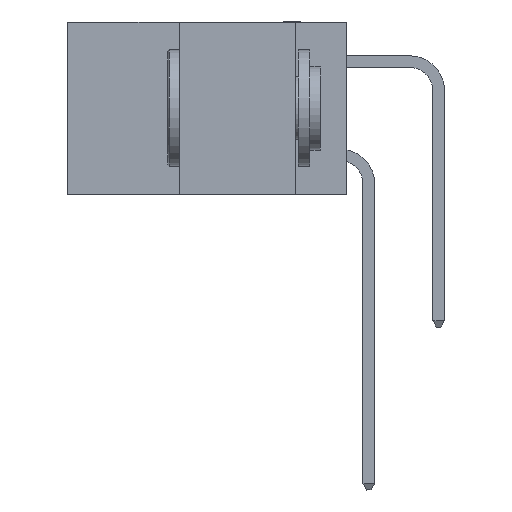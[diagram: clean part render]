
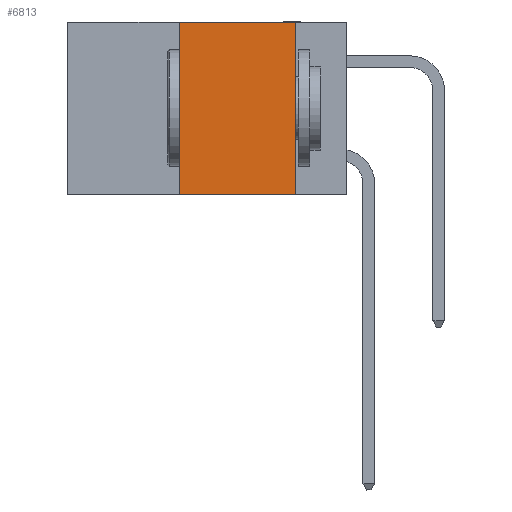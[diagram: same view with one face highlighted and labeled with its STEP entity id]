
A CAD part, left-side view. The second image highlights one B-rep face of the part: STEP entity #6813.
In plain terms, the highlighted planar face has unit normal (-1, 0, 0).
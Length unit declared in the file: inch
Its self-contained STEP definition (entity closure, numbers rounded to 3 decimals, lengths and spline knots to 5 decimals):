
#125 = EDGE_CURVE ( 'NONE', #14238, #33200, #35352, .T. ) ;
#532 = CARTESIAN_POINT ( 'NONE',  ( 0., 0.6, 0. ) ) ;
#647 = DIRECTION ( 'NONE',  ( 0., 0., -1. ) ) ;
#1211 = EDGE_LOOP ( 'NONE', ( #28607, #25209, #31138, #18155 ) ) ;
#2256 = LINE ( 'NONE', #3740, #25788 ) ;
#3740 = CARTESIAN_POINT ( 'NONE',  ( 0., 0.36, 0. ) ) ;
#4098 = EDGE_CURVE ( 'NONE', #16707, #33200, #16321, .T. ) ;
#5903 = VECTOR ( 'NONE', #12400, 39.37008 ) ;
#6072 = PLANE ( 'NONE',  #8083 ) ;
#6355 = DIRECTION ( 'NONE',  ( 0., 0., 1. ) ) ;
#6497 = VECTOR ( 'NONE', #10852, 39.37008 ) ;
#6813 = ADVANCED_FACE ( 'NONE', ( #23195 ), #6072, .F. ) ;
#8083 = AXIS2_PLACEMENT_3D ( 'NONE', #532, #8919, #647 ) ;
#8919 = DIRECTION ( 'NONE',  ( 1., 0., 0. ) ) ;
#10130 = CARTESIAN_POINT ( 'NONE',  ( 0., 0.6, 0. ) ) ;
#10710 = EDGE_CURVE ( 'NONE', #28517, #16707, #28881, .T. ) ;
#10852 = DIRECTION ( 'NONE',  ( 0., 0., -1. ) ) ;
#12400 = DIRECTION ( 'NONE',  ( 0., -1., 0. ) ) ;
#14238 = VERTEX_POINT ( 'NONE', #29024 ) ;
#16321 = LINE ( 'NONE', #32690, #6497 ) ;
#16685 = CARTESIAN_POINT ( 'NONE',  ( 0., 0.36, 0. ) ) ;
#16707 = VERTEX_POINT ( 'NONE', #31002 ) ;
#18155 = ORIENTED_EDGE ( 'NONE', *, *, #125, .T. ) ;
#18355 = DIRECTION ( 'NONE',  ( 0., -1., 0. ) ) ;
#23195 = FACE_OUTER_BOUND ( 'NONE', #1211, .T. ) ;
#23327 = VECTOR ( 'NONE', #18355, 39.37008 ) ;
#25209 = ORIENTED_EDGE ( 'NONE', *, *, #10710, .F. ) ;
#25788 = VECTOR ( 'NONE', #6355, 39.37008 ) ;
#26447 = CARTESIAN_POINT ( 'NONE',  ( 0., 0.11, -0.37 ) ) ;
#26882 = CARTESIAN_POINT ( 'NONE',  ( 0., 0.6, -0.37 ) ) ;
#28517 = VERTEX_POINT ( 'NONE', #16685 ) ;
#28607 = ORIENTED_EDGE ( 'NONE', *, *, #4098, .F. ) ;
#28881 = LINE ( 'NONE', #10130, #23327 ) ;
#29024 = CARTESIAN_POINT ( 'NONE',  ( 0., 0.36, -0.37 ) ) ;
#31002 = CARTESIAN_POINT ( 'NONE',  ( 0., 0.11, 0. ) ) ;
#31138 = ORIENTED_EDGE ( 'NONE', *, *, #31900, .F. ) ;
#31900 = EDGE_CURVE ( 'NONE', #14238, #28517, #2256, .T. ) ;
#32690 = CARTESIAN_POINT ( 'NONE',  ( 0., 0.11, 0. ) ) ;
#33200 = VERTEX_POINT ( 'NONE', #26447 ) ;
#35352 = LINE ( 'NONE', #26882, #5903 ) ;
